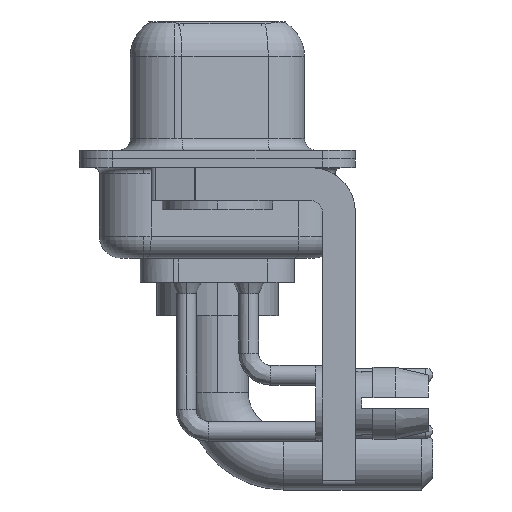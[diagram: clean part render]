
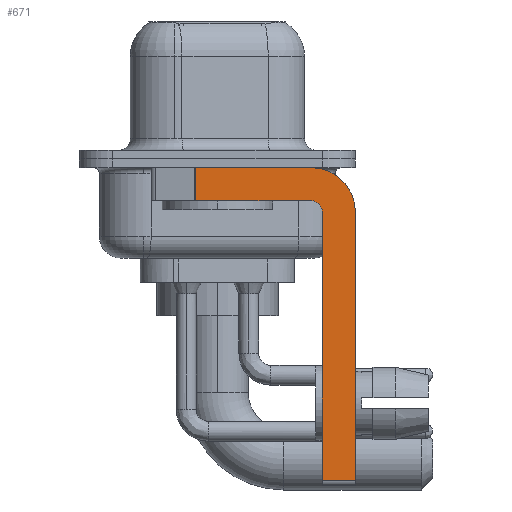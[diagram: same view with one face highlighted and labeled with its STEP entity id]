
A CAD part, left-side view. The second image highlights one B-rep face of the part: STEP entity #671.
In plain terms, the highlighted planar face has unit normal (-1, 0, 0).
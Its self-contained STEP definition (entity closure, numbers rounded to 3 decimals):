
#91 = DIRECTION ( 'NONE',  ( 0., 0., 1. ) ) ;
#353 = DIRECTION ( 'NONE',  ( 0., -1., 0. ) ) ;
#400 = CARTESIAN_POINT ( 'NONE',  ( -2.9, -4.75, -14.8 ) ) ;
#671 = ADVANCED_FACE ( 'NONE', ( #21053 ), #14203, .F. ) ;
#818 = LINE ( 'NONE', #12110, #2958 ) ;
#924 = LINE ( 'NONE', #16794, #11624 ) ;
#1433 = CARTESIAN_POINT ( 'NONE',  ( -2.9, -4.25, -2.4 ) ) ;
#1578 = EDGE_LOOP ( 'NONE', ( #18961, #14902, #8884, #8443, #15113, #20952, #16560, #6961 ) ) ;
#1994 = DIRECTION ( 'NONE',  ( 0., 0., -1. ) ) ;
#2774 = CIRCLE ( 'NONE', #6844, 0.5 ) ;
#2958 = VECTOR ( 'NONE', #1994, 1000. ) ;
#3266 = VERTEX_POINT ( 'NONE', #15329 ) ;
#3769 = EDGE_CURVE ( 'NONE', #11408, #15534, #924, .T. ) ;
#3805 = VECTOR ( 'NONE', #10821, 1000. ) ;
#5507 = DIRECTION ( 'NONE',  ( 0., -1., 0. ) ) ;
#5718 = LINE ( 'NONE', #10920, #3805 ) ;
#6086 = DIRECTION ( 'NONE',  ( 0., 1., 0. ) ) ;
#6127 = DIRECTION ( 'NONE',  ( -1., 0., 0. ) ) ;
#6203 = EDGE_CURVE ( 'NONE', #13729, #9465, #20598, .T. ) ;
#6844 = AXIS2_PLACEMENT_3D ( 'NONE', #17206, #6127, #20953 ) ;
#6961 = ORIENTED_EDGE ( 'NONE', *, *, #20530, .F. ) ;
#7784 = EDGE_CURVE ( 'NONE', #11408, #17028, #8170, .T. ) ;
#8170 = LINE ( 'NONE', #400, #15775 ) ;
#8443 = ORIENTED_EDGE ( 'NONE', *, *, #20131, .F. ) ;
#8864 = AXIS2_PLACEMENT_3D ( 'NONE', #9678, #11293, #18982 ) ;
#8884 = ORIENTED_EDGE ( 'NONE', *, *, #6203, .F. ) ;
#8970 = EDGE_CURVE ( 'NONE', #16510, #3266, #9929, .T. ) ;
#9251 = VECTOR ( 'NONE', #6086, 1000. ) ;
#9302 = DIRECTION ( 'NONE',  ( 1., 0., 0. ) ) ;
#9465 = VERTEX_POINT ( 'NONE', #9685 ) ;
#9604 = CARTESIAN_POINT ( 'NONE',  ( -2.9, 0.978, -0.4 ) ) ;
#9678 = CARTESIAN_POINT ( 'NONE',  ( -2.9, -4.25, -2.4 ) ) ;
#9685 = CARTESIAN_POINT ( 'NONE',  ( -2.9, 0.978, -1.9 ) ) ;
#9717 = DIRECTION ( 'NONE',  ( 0., 0., -1. ) ) ;
#9813 = AXIS2_PLACEMENT_3D ( 'NONE', #1433, #9302, #9717 ) ;
#9929 = LINE ( 'NONE', #16530, #11423 ) ;
#10536 = EDGE_CURVE ( 'NONE', #16510, #9465, #818, .T. ) ;
#10821 = DIRECTION ( 'NONE',  ( 0., 0., -1. ) ) ;
#10920 = CARTESIAN_POINT ( 'NONE',  ( -2.9, -6.25, -2.4 ) ) ;
#11196 = CARTESIAN_POINT ( 'NONE',  ( -2.9, -4.25, -1.9 ) ) ;
#11293 = DIRECTION ( 'NONE',  ( 1., 0., 0. ) ) ;
#11408 = VERTEX_POINT ( 'NONE', #14647 ) ;
#11423 = VECTOR ( 'NONE', #353, 1000. ) ;
#11508 = CARTESIAN_POINT ( 'NONE',  ( -2.9, -4.75, -2.4 ) ) ;
#11624 = VECTOR ( 'NONE', #5507, 1000. ) ;
#11637 = CIRCLE ( 'NONE', #8864, 2. ) ;
#12110 = CARTESIAN_POINT ( 'NONE',  ( -2.9, 0.978, -1.9 ) ) ;
#13729 = VERTEX_POINT ( 'NONE', #11196 ) ;
#14203 = PLANE ( 'NONE',  #9813 ) ;
#14647 = CARTESIAN_POINT ( 'NONE',  ( -2.9, -4.75, -14.55 ) ) ;
#14902 = ORIENTED_EDGE ( 'NONE', *, *, #10536, .T. ) ;
#15113 = ORIENTED_EDGE ( 'NONE', *, *, #7784, .F. ) ;
#15329 = CARTESIAN_POINT ( 'NONE',  ( -2.9, -4.25, -0.4 ) ) ;
#15534 = VERTEX_POINT ( 'NONE', #17466 ) ;
#15775 = VECTOR ( 'NONE', #91, 1000. ) ;
#16510 = VERTEX_POINT ( 'NONE', #9604 ) ;
#16527 = VERTEX_POINT ( 'NONE', #20931 ) ;
#16530 = CARTESIAN_POINT ( 'NONE',  ( -2.9, 3., -0.4 ) ) ;
#16560 = ORIENTED_EDGE ( 'NONE', *, *, #20008, .F. ) ;
#16794 = CARTESIAN_POINT ( 'NONE',  ( -2.9, -4.25, -14.55 ) ) ;
#17028 = VERTEX_POINT ( 'NONE', #11508 ) ;
#17206 = CARTESIAN_POINT ( 'NONE',  ( -2.9, -4.25, -2.4 ) ) ;
#17466 = CARTESIAN_POINT ( 'NONE',  ( -2.9, -6.25, -14.55 ) ) ;
#18961 = ORIENTED_EDGE ( 'NONE', *, *, #8970, .F. ) ;
#18982 = DIRECTION ( 'NONE',  ( 0., 0., -1. ) ) ;
#20008 = EDGE_CURVE ( 'NONE', #16527, #15534, #5718, .T. ) ;
#20131 = EDGE_CURVE ( 'NONE', #17028, #13729, #2774, .T. ) ;
#20530 = EDGE_CURVE ( 'NONE', #3266, #16527, #11637, .T. ) ;
#20598 = LINE ( 'NONE', #20699, #9251 ) ;
#20699 = CARTESIAN_POINT ( 'NONE',  ( -2.9, -4.25, -1.9 ) ) ;
#20931 = CARTESIAN_POINT ( 'NONE',  ( -2.9, -6.25, -2.4 ) ) ;
#20952 = ORIENTED_EDGE ( 'NONE', *, *, #3769, .T. ) ;
#20953 = DIRECTION ( 'NONE',  ( 0., 0., 1. ) ) ;
#21053 = FACE_OUTER_BOUND ( 'NONE', #1578, .T. ) ;
